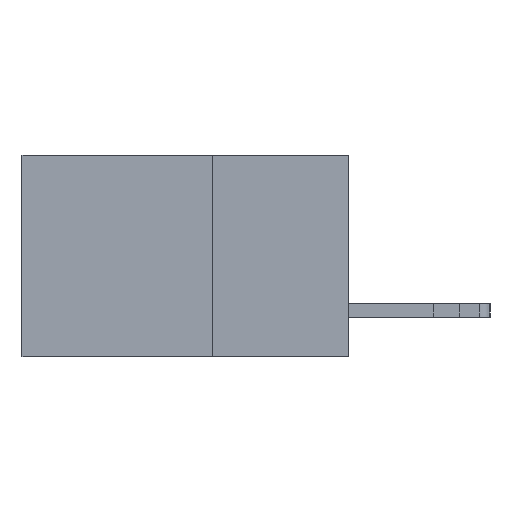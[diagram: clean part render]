
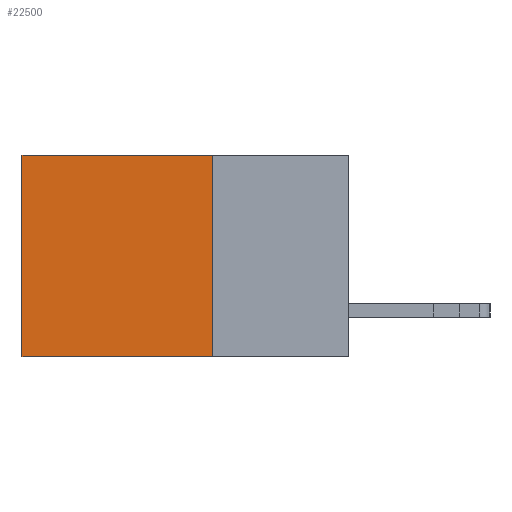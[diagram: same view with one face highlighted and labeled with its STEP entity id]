
A CAD part, left-side view. The second image highlights one B-rep face of the part: STEP entity #22500.
In plain terms, the highlighted planar face has unit normal (-1, 0, 0).
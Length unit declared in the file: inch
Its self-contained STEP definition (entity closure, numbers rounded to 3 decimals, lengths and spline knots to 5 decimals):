
#980 = ORIENTED_EDGE ( 'NONE', *, *, #13235, .F. ) ;
#1101 = ORIENTED_EDGE ( 'NONE', *, *, #18014, .T. ) ;
#1822 = PLANE ( 'NONE',  #2901 ) ;
#1960 = VERTEX_POINT ( 'NONE', #11187 ) ;
#2901 = AXIS2_PLACEMENT_3D ( 'NONE', #19970, #8002, #21975 ) ;
#3984 = VERTEX_POINT ( 'NONE', #5171 ) ;
#4113 = ORIENTED_EDGE ( 'NONE', *, *, #14340, .T. ) ;
#4131 = DIRECTION ( 'NONE',  ( 0., 0., -1. ) ) ;
#4486 = LINE ( 'NONE', #11508, #19210 ) ;
#5171 = CARTESIAN_POINT ( 'NONE',  ( 0.2615, 0.25, 0. ) ) ;
#8002 = DIRECTION ( 'NONE',  ( 1., 0., 0. ) ) ;
#9311 = DIRECTION ( 'NONE',  ( 0., 1., 0. ) ) ;
#9989 = LINE ( 'NONE', #10126, #19996 ) ;
#10126 = CARTESIAN_POINT ( 'NONE',  ( 0.2615, 0.6, -0.37 ) ) ;
#11048 = CARTESIAN_POINT ( 'NONE',  ( 0.2615, 0.25, 0. ) ) ;
#11187 = CARTESIAN_POINT ( 'NONE',  ( 0.2615, 0.6, 0. ) ) ;
#11508 = CARTESIAN_POINT ( 'NONE',  ( 0.2615, 0.25, -0.37 ) ) ;
#12626 = LINE ( 'NONE', #11048, #17282 ) ;
#13222 = CARTESIAN_POINT ( 'NONE',  ( 0.2615, 0.25, -0.37 ) ) ;
#13235 = EDGE_CURVE ( 'NONE', #3984, #22519, #4486, .T. ) ;
#14340 = EDGE_CURVE ( 'NONE', #3984, #1960, #12626, .T. ) ;
#15418 = DIRECTION ( 'NONE',  ( 0., 0., -1. ) ) ;
#15991 = CARTESIAN_POINT ( 'NONE',  ( 0.2615, 0.25, -0.37 ) ) ;
#16348 = VECTOR ( 'NONE', #9311, 39.37008 ) ;
#16968 = LINE ( 'NONE', #13222, #16348 ) ;
#17282 = VECTOR ( 'NONE', #21014, 39.37008 ) ;
#18014 = EDGE_CURVE ( 'NONE', #1960, #22475, #9989, .T. ) ;
#18036 = ORIENTED_EDGE ( 'NONE', *, *, #20921, .F. ) ;
#19210 = VECTOR ( 'NONE', #15418, 39.37008 ) ;
#19782 = CARTESIAN_POINT ( 'NONE',  ( 0.2615, 0.6, -0.37 ) ) ;
#19970 = CARTESIAN_POINT ( 'NONE',  ( 0.2615, 0.25, -0.37 ) ) ;
#19996 = VECTOR ( 'NONE', #4131, 39.37008 ) ;
#20921 = EDGE_CURVE ( 'NONE', #22519, #22475, #16968, .T. ) ;
#21014 = DIRECTION ( 'NONE',  ( 0., 1., 0. ) ) ;
#21975 = DIRECTION ( 'NONE',  ( 0., 0., -1. ) ) ;
#22475 = VERTEX_POINT ( 'NONE', #19782 ) ;
#22500 = ADVANCED_FACE ( 'NONE', ( #25173 ), #1822, .F. ) ;
#22519 = VERTEX_POINT ( 'NONE', #15991 ) ;
#25173 = FACE_OUTER_BOUND ( 'NONE', #25221, .T. ) ;
#25221 = EDGE_LOOP ( 'NONE', ( #1101, #18036, #980, #4113 ) ) ;
